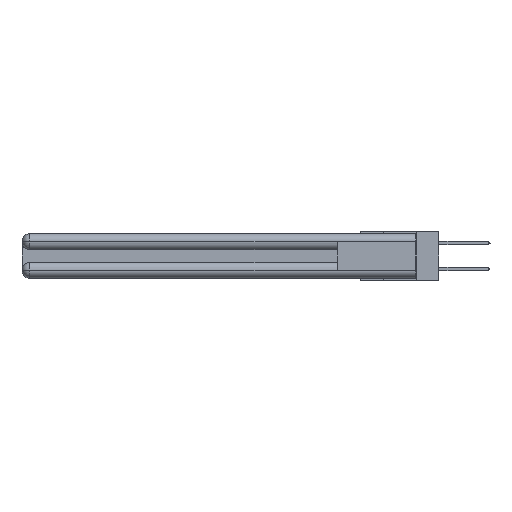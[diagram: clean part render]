
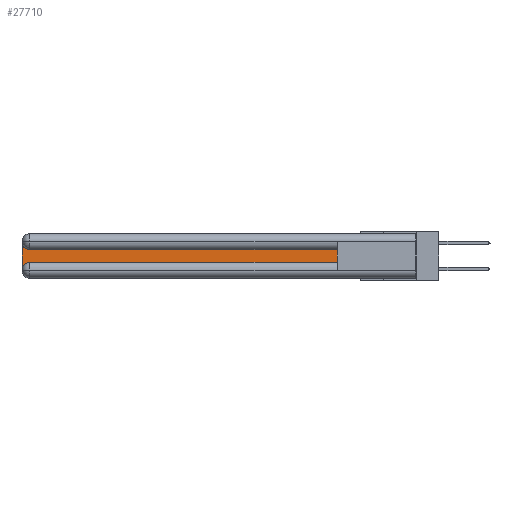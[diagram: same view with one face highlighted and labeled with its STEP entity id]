
A CAD part, left-side view. The second image highlights one B-rep face of the part: STEP entity #27710.
In plain terms, the highlighted planar face has unit normal (-1, 0, 0).
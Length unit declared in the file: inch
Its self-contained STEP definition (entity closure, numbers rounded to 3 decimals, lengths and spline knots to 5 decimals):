
#97 = AXIS2_PLACEMENT_3D ( 'NONE', #848, #17549, #8053 ) ;
#414 = AXIS2_PLACEMENT_3D ( 'NONE', #17296, #19594, #5588 ) ;
#527 = DIRECTION ( 'NONE',  ( 0., 0., 1. ) ) ;
#727 = CARTESIAN_POINT ( 'NONE',  ( 0.075, 0.6, -0.2175 ) ) ;
#848 = CARTESIAN_POINT ( 'NONE',  ( 0.075, 2.94, -0.2775 ) ) ;
#1040 = LINE ( 'NONE', #9628, #18611 ) ;
#3199 = VERTEX_POINT ( 'NONE', #3468 ) ;
#3223 = EDGE_CURVE ( 'NONE', #7287, #9951, #3275, .T. ) ;
#3275 = LINE ( 'NONE', #4586, #24455 ) ;
#3468 = CARTESIAN_POINT ( 'NONE',  ( 0.075, 2.94, -0.2175 ) ) ;
#3723 = ORIENTED_EDGE ( 'NONE', *, *, #20643, .T. ) ;
#4263 = CARTESIAN_POINT ( 'NONE',  ( 0.075, 3., -0.2775 ) ) ;
#4432 = VERTEX_POINT ( 'NONE', #14692 ) ;
#4586 = CARTESIAN_POINT ( 'NONE',  ( 0.075, 3., -0.2175 ) ) ;
#5084 = DIRECTION ( 'NONE',  ( 0., 0., -1. ) ) ;
#5588 = DIRECTION ( 'NONE',  ( 0., 0., -1. ) ) ;
#6724 = CARTESIAN_POINT ( 'NONE',  ( 0.075, 0.6, -0.1225 ) ) ;
#6805 = EDGE_CURVE ( 'NONE', #9951, #3199, #24752, .T. ) ;
#7287 = VERTEX_POINT ( 'NONE', #29668 ) ;
#7629 = VERTEX_POINT ( 'NONE', #29906 ) ;
#8053 = DIRECTION ( 'NONE',  ( 0., 0., -1. ) ) ;
#8064 = LINE ( 'NONE', #727, #13967 ) ;
#8381 = PLANE ( 'NONE',  #16369 ) ;
#9628 = CARTESIAN_POINT ( 'NONE',  ( 0.075, 0.6, -0.2175 ) ) ;
#9951 = VERTEX_POINT ( 'NONE', #4263 ) ;
#10651 = DIRECTION ( 'NONE',  ( 0., 0., -1. ) ) ;
#11710 = ORIENTED_EDGE ( 'NONE', *, *, #13635, .T. ) ;
#13070 = EDGE_CURVE ( 'NONE', #7629, #7287, #26593, .T. ) ;
#13298 = EDGE_CURVE ( 'NONE', #4432, #14978, #8064, .T. ) ;
#13497 = FACE_OUTER_BOUND ( 'NONE', #26873, .T. ) ;
#13635 = EDGE_CURVE ( 'NONE', #14978, #7629, #23684, .T. ) ;
#13967 = VECTOR ( 'NONE', #527, 39.37008 ) ;
#14039 = DIRECTION ( 'NONE',  ( 0., -1., 0. ) ) ;
#14118 = ORIENTED_EDGE ( 'NONE', *, *, #13298, .T. ) ;
#14692 = CARTESIAN_POINT ( 'NONE',  ( 0.075, 0.6, -0.2175 ) ) ;
#14978 = VERTEX_POINT ( 'NONE', #18476 ) ;
#16369 = AXIS2_PLACEMENT_3D ( 'NONE', #24436, #29300, #10651 ) ;
#17203 = ORIENTED_EDGE ( 'NONE', *, *, #13070, .T. ) ;
#17296 = CARTESIAN_POINT ( 'NONE',  ( 0.075, 2.94, -0.0625 ) ) ;
#17549 = DIRECTION ( 'NONE',  ( 1., 0., 0. ) ) ;
#18476 = CARTESIAN_POINT ( 'NONE',  ( 0.075, 0.6, -0.1225 ) ) ;
#18611 = VECTOR ( 'NONE', #14039, 39.37008 ) ;
#19010 = ORIENTED_EDGE ( 'NONE', *, *, #3223, .T. ) ;
#19594 = DIRECTION ( 'NONE',  ( 1., 0., 0. ) ) ;
#20643 = EDGE_CURVE ( 'NONE', #3199, #4432, #1040, .T. ) ;
#23014 = DIRECTION ( 'NONE',  ( 0., 1., 0. ) ) ;
#23684 = LINE ( 'NONE', #6724, #29135 ) ;
#24436 = CARTESIAN_POINT ( 'NONE',  ( 0.075, 3., -0.1225 ) ) ;
#24455 = VECTOR ( 'NONE', #5084, 39.37008 ) ;
#24752 = CIRCLE ( 'NONE', #97, 0.06 ) ;
#26593 = CIRCLE ( 'NONE', #414, 0.06 ) ;
#26873 = EDGE_LOOP ( 'NONE', ( #11710, #17203, #19010, #27410, #3723, #14118 ) ) ;
#27410 = ORIENTED_EDGE ( 'NONE', *, *, #6805, .T. ) ;
#27710 = ADVANCED_FACE ( 'NONE', ( #13497 ), #8381, .F. ) ;
#29135 = VECTOR ( 'NONE', #23014, 39.37008 ) ;
#29300 = DIRECTION ( 'NONE',  ( 1., 0., 0. ) ) ;
#29668 = CARTESIAN_POINT ( 'NONE',  ( 0.075, 3., -0.0625 ) ) ;
#29906 = CARTESIAN_POINT ( 'NONE',  ( 0.075, 2.94, -0.1225 ) ) ;
